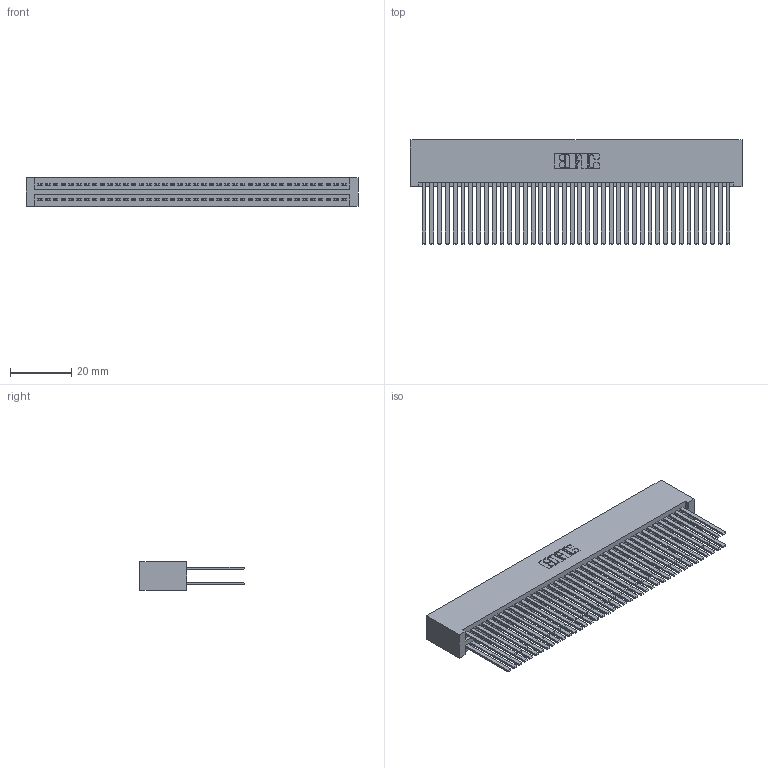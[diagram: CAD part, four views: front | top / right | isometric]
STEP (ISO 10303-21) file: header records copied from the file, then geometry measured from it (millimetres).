
FILE_DESCRIPTION (( 'STEP AP203' ), '1' );
FILE_NAME ('345-080-544-201.STEP', '2018-10-03T18:27:31', ( '' ), ( '' ), 'SwSTEP 2.0', 'SolidWorks 2016', '' );
FILE_SCHEMA (( 'CONFIG_CONTROL_DESIGN' ));
Length unit declared in the file: inch
Products named in the file (3): 345-080-544-201; 345-292-001_345-293-144; 345 Part_No Mounting Lugs
Assembly tree (81 placements, depth 2):
  345-080-544-201
    345 Part_No Mounting Lugs
    345-292-001_345-293-144  x80
Bounding box: 108.2 x 33.96 x 9.4 mm (x, y, z)
Volume: 12229.8 mm3; surface area: 21629.2 mm2
Topology: 81 solids, 81 shells, 3638 faces, 10797 edges, 7090 vertices
Faces by surface type: plane 2396, cylinder 1242
Entity records: 31193 total; most frequent: CARTESIAN_POINT 5228, ORIENTED_EDGE 5162, DIRECTION 4605, EDGE_CURVE 2581, LINE 2301, VECTOR 2301, VERTEX_POINT 1718, AXIS2_PLACEMENT_3D 1152
